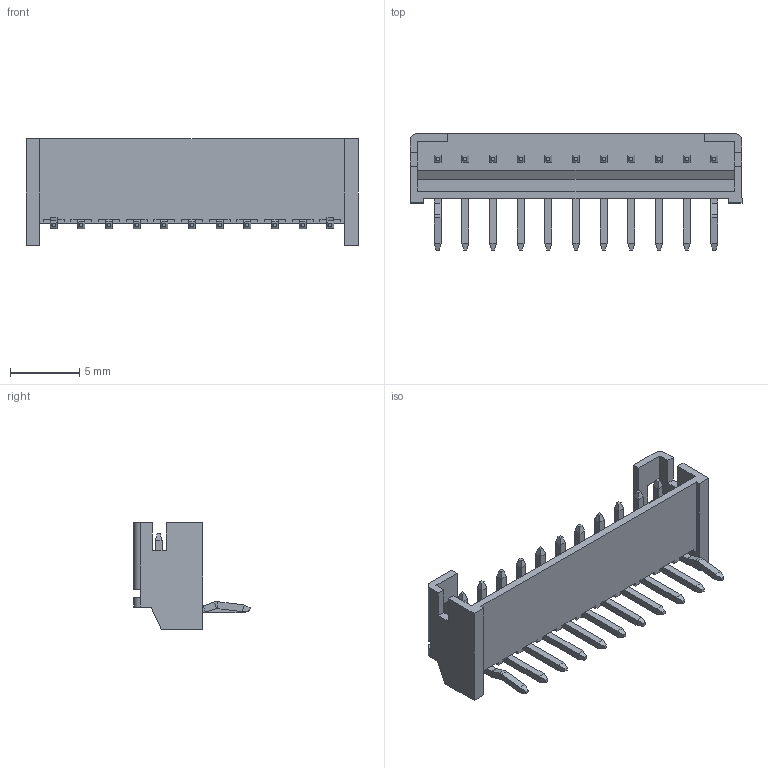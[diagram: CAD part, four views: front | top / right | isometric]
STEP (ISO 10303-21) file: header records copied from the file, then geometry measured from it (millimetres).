
FILE_DESCRIPTION (( 'STEP AP203' ), '1' );
FILE_NAME ('140-511-415-000.STEP', '2020-03-31T19:45:02', ( '' ), ( '' ), 'SwSTEP 2.0', 'SolidWorks 2016', '' );
FILE_SCHEMA (( 'CONFIG_CONTROL_DESIGN' ));
Length unit declared in the file: millimetre
Products named in the file (4): RA Contact_Kink; 140-511-415-000; RA Housing_511; RA Contact_Str
Assembly tree (12 placements, depth 2):
  140-511-415-000
    RA Housing_511
    RA Contact_Kink  x2
    RA Contact_Str  x9
Bounding box: 24 x 8.41 x 7.7 mm (x, y, z)
Volume: 279.1 mm3; surface area: 1029 mm2
Topology: 12 solids, 12 shells, 409 faces, 949 edges, 562 vertices
Faces by surface type: plane 375, cylinder 34
Entity records: 6657 total; most frequent: CARTESIAN_POINT 1061, ORIENTED_EDGE 1042, DIRECTION 965, EDGE_CURVE 521, VECTOR 497, LINE 497, VERTEX_POINT 330, AXIS2_PLACEMENT_3D 234
